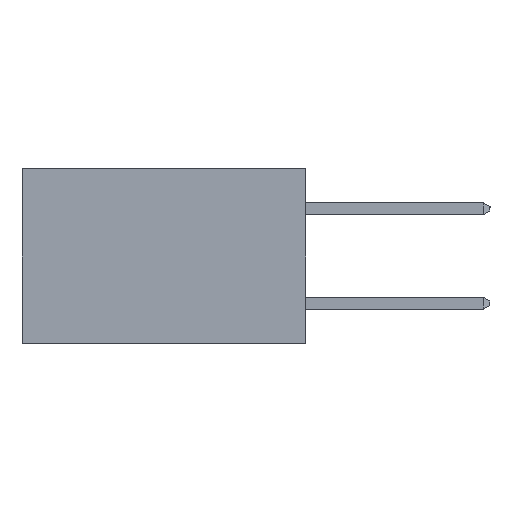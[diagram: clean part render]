
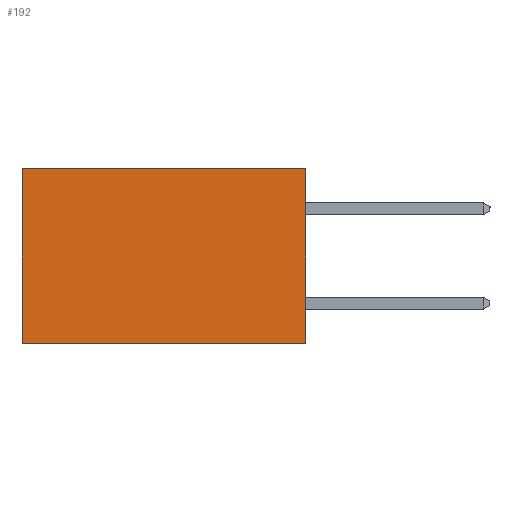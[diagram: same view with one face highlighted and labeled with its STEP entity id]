
A CAD part, left-side view. The second image highlights one B-rep face of the part: STEP entity #192.
In plain terms, the highlighted planar face has unit normal (-1, 0, 0).
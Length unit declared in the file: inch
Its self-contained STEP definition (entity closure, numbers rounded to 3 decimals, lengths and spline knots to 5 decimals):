
#139 = DIRECTION ( 'NONE',  ( 0., 0., -1. ) ) ;
#192 = ADVANCED_FACE ( 'NONE', ( #12868 ), #12427, .F. ) ;
#981 = CARTESIAN_POINT ( 'NONE',  ( 0.2615, 0., -0.37 ) ) ;
#1131 = DIRECTION ( 'NONE',  ( 0., 0., -1. ) ) ;
#1269 = EDGE_CURVE ( 'NONE', #15046, #15977, #13874, .T. ) ;
#1539 = ORIENTED_EDGE ( 'NONE', *, *, #1269, .T. ) ;
#1694 = EDGE_LOOP ( 'NONE', ( #3172, #8886, #7098, #1539 ) ) ;
#1781 = CARTESIAN_POINT ( 'NONE',  ( 0.2615, 0.6, -0.37 ) ) ;
#3172 = ORIENTED_EDGE ( 'NONE', *, *, #14989, .T. ) ;
#3577 = CARTESIAN_POINT ( 'NONE',  ( 0.2615, 0.6, 0. ) ) ;
#4737 = CARTESIAN_POINT ( 'NONE',  ( 0.2615, 0., 0. ) ) ;
#5029 = VECTOR ( 'NONE', #10304, 39.37008 ) ;
#5173 = VERTEX_POINT ( 'NONE', #14329 ) ;
#5342 = CARTESIAN_POINT ( 'NONE',  ( 0.2615, 0., 0. ) ) ;
#5873 = LINE ( 'NONE', #981, #12728 ) ;
#6020 = EDGE_CURVE ( 'NONE', #5173, #12874, #6421, .T. ) ;
#6193 = VECTOR ( 'NONE', #9617, 39.37008 ) ;
#6421 = LINE ( 'NONE', #10118, #8985 ) ;
#7098 = ORIENTED_EDGE ( 'NONE', *, *, #8549, .F. ) ;
#8091 = AXIS2_PLACEMENT_3D ( 'NONE', #10359, #12703, #139 ) ;
#8549 = EDGE_CURVE ( 'NONE', #15046, #5173, #5873, .T. ) ;
#8886 = ORIENTED_EDGE ( 'NONE', *, *, #6020, .F. ) ;
#8985 = VECTOR ( 'NONE', #15074, 39.37008 ) ;
#9617 = DIRECTION ( 'NONE',  ( 0., 1., 0. ) ) ;
#10118 = CARTESIAN_POINT ( 'NONE',  ( 0.2615, 0., -0.37 ) ) ;
#10304 = DIRECTION ( 'NONE',  ( 0., 0., -1. ) ) ;
#10359 = CARTESIAN_POINT ( 'NONE',  ( 0.2615, 0., -0.37 ) ) ;
#11786 = CARTESIAN_POINT ( 'NONE',  ( 0.2615, 0.6, -0.37 ) ) ;
#12427 = PLANE ( 'NONE',  #8091 ) ;
#12703 = DIRECTION ( 'NONE',  ( 1., 0., 0. ) ) ;
#12728 = VECTOR ( 'NONE', #1131, 39.37008 ) ;
#12868 = FACE_OUTER_BOUND ( 'NONE', #1694, .T. ) ;
#12874 = VERTEX_POINT ( 'NONE', #1781 ) ;
#13874 = LINE ( 'NONE', #4737, #6193 ) ;
#14130 = LINE ( 'NONE', #11786, #5029 ) ;
#14329 = CARTESIAN_POINT ( 'NONE',  ( 0.2615, 0., -0.37 ) ) ;
#14989 = EDGE_CURVE ( 'NONE', #15977, #12874, #14130, .T. ) ;
#15046 = VERTEX_POINT ( 'NONE', #5342 ) ;
#15074 = DIRECTION ( 'NONE',  ( 0., 1., 0. ) ) ;
#15977 = VERTEX_POINT ( 'NONE', #3577 ) ;
